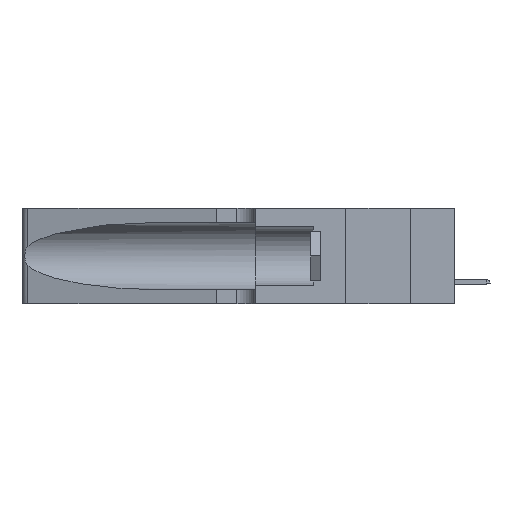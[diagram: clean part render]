
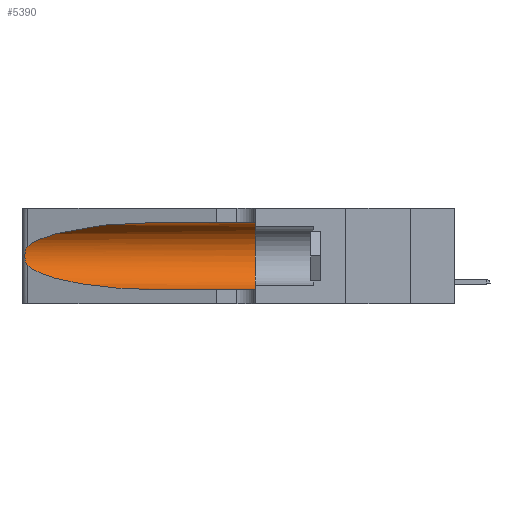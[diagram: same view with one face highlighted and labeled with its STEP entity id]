
A CAD part, left-side view. The second image highlights one B-rep face of the part: STEP entity #5390.
In plain terms, the highlighted cylindrical face has radius 3.308 mm (diameter 6.617 mm), a partial arc.
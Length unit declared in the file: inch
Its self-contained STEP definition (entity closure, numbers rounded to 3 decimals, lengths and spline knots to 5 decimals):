
#290 = CARTESIAN_POINT ( 'NONE',  ( 0.1305, 0.72297, 0.31525 ) ) ;
#758 = DIRECTION ( 'NONE',  ( 0., 0., 1. ) ) ;
#1511 = CARTESIAN_POINT ( 'NONE',  ( 0.25787, 1.23484, 0.2124 ) ) ;
#2479 = VERTEX_POINT ( 'NONE', #25399 ) ;
#2814 = DIRECTION ( 'NONE',  ( 0., -1., 0. ) ) ;
#3472 = DIRECTION ( 'NONE',  ( 0., 1., 0. ) ) ;
#3632 = ORIENTED_EDGE ( 'NONE', *, *, #14990, .T. ) ;
#4220 = CARTESIAN_POINT ( 'NONE',  ( 0.25856, 1.23593, 0.16098 ) ) ;
#5390 = ADVANCED_FACE ( 'NONE', ( #10882 ), #11783, .F. ) ;
#5573 = EDGE_LOOP ( 'NONE', ( #14647, #34118, #3632, #6699, #36847, #7488 ) ) ;
#5794 = LINE ( 'NONE', #29427, #13651 ) ;
#6699 = ORIENTED_EDGE ( 'NONE', *, *, #7355, .T. ) ;
#7143 = CARTESIAN_POINT ( 'NONE',  ( 0.26075, 1.23896, 0.19203 ) ) ;
#7355 = EDGE_CURVE ( 'NONE', #11016, #2479, #20298, .T. ) ;
#7488 = ORIENTED_EDGE ( 'NONE', *, *, #14777, .F. ) ;
#7536 = EDGE_CURVE ( 'NONE', #10165, #36781, #24513, .T. ) ;
#8660 = DIRECTION ( 'NONE',  ( 0., 0., -1. ) ) ;
#8939 = EDGE_CURVE ( 'NONE', #36781, #21660, #22074, .T. ) ;
#10009 = CARTESIAN_POINT ( 'NONE',  ( 0.25487, 1.22718, 0.22369 ) ) ;
#10065 = CARTESIAN_POINT ( 'NONE',  ( 0.26018, 1.23835, 0.19895 ) ) ;
#10165 = VERTEX_POINT ( 'NONE', #13570 ) ;
#10266 = CARTESIAN_POINT ( 'NONE',  ( 0.26017, 1.23833, 0.17102 ) ) ;
#10743 = CARTESIAN_POINT ( 'NONE',  ( 0.1305, 0.72297, 0.05475 ) ) ;
#10882 = FACE_OUTER_BOUND ( 'NONE', #5573, .T. ) ;
#11016 = VERTEX_POINT ( 'NONE', #10743 ) ;
#11783 = CYLINDRICAL_SURFACE ( 'NONE', #23109, 0.13025 ) ;
#12361 = CARTESIAN_POINT ( 'NONE',  ( 0.2373, 1.15595, 0.28018 ) ) ;
#13380 = CARTESIAN_POINT ( 'NONE',  ( 0.25555, 1.22993, 0.14849 ) ) ;
#13570 = CARTESIAN_POINT ( 'NONE',  ( 0.1305, 0.72297, 0.31525 ) ) ;
#13651 = VECTOR ( 'NONE', #14919, 39.37008 ) ;
#14504 = CARTESIAN_POINT ( 'NONE',  ( 0.1305, 1.61858, 0.05475 ) ) ;
#14647 = ORIENTED_EDGE ( 'NONE', *, *, #7536, .T. ) ;
#14688 = VERTEX_POINT ( 'NONE', #16323 ) ;
#14751 = CARTESIAN_POINT ( 'NONE',  ( 0.1305, 0.35, 0.185 ) ) ;
#14755 = AXIS2_PLACEMENT_3D ( 'NONE', #14751, #3472, #758 ) ;
#14777 = EDGE_CURVE ( 'NONE', #10165, #14688, #5794, .T. ) ;
#14919 = DIRECTION ( 'NONE',  ( 0., -1., 0. ) ) ;
#14990 = EDGE_CURVE ( 'NONE', #21660, #11016, #15143, .T. ) ;
#15109 = CARTESIAN_POINT ( 'NONE',  ( 0.25487, 1.22718, 0.22369 ) ) ;
#15143 =( BOUNDED_CURVE ( )  B_SPLINE_CURVE ( 3, ( #33874, #16657, #16080, #37141 ),
 .UNSPECIFIED., .F., .T. ) 
 B_SPLINE_CURVE_WITH_KNOTS ( ( 4, 4 ),
 ( 3.44316, 4.71239 ),
 .UNSPECIFIED. ) 
 CURVE ( )  GEOMETRIC_REPRESENTATION_ITEM ( )  RATIONAL_B_SPLINE_CURVE ( ( 1., 0.87, 0.87, 1. ) ) 
 REPRESENTATION_ITEM ( '' )  );
#16080 = CARTESIAN_POINT ( 'NONE',  ( 0.18966, 0.96281, 0.05475 ) ) ;
#16098 = CARTESIAN_POINT ( 'NONE',  ( 0.25487, 1.22718, 0.14631 ) ) ;
#16323 = CARTESIAN_POINT ( 'NONE',  ( 0.1305, 0.35, 0.31525 ) ) ;
#16657 = CARTESIAN_POINT ( 'NONE',  ( 0.2373, 1.15595, 0.08982 ) ) ;
#18933 = CARTESIAN_POINT ( 'NONE',  ( 0.18966, 0.96281, 0.31525 ) ) ;
#19383 = CARTESIAN_POINT ( 'NONE',  ( 0.25789, 1.23486, 0.15765 ) ) ;
#19882 = CARTESIAN_POINT ( 'NONE',  ( 0.25487, 1.22718, 0.14631 ) ) ;
#20254 = VECTOR ( 'NONE', #2814, 39.37008 ) ;
#20298 = LINE ( 'NONE', #14504, #20254 ) ;
#21132 = CARTESIAN_POINT ( 'NONE',  ( 0.25487, 1.22718, 0.22369 ) ) ;
#21660 = VERTEX_POINT ( 'NONE', #19882 ) ;
#22074 = B_SPLINE_CURVE_WITH_KNOTS ( 'NONE', 3,
 ( #21132, #29441, #30411, #1511, #36590, #10065, #7143, #33889, #10266, #4220, #19383, #30987, #13380, #16098 ),
 .UNSPECIFIED., .F., .F.,
 ( 4, 2, 2, 2, 2, 2, 4 ),
 ( 0., 0.00027, 0.00053, 0.00107, 0.0016, 0.00187, 0.00214 ),
 .UNSPECIFIED. ) ;
#23109 = AXIS2_PLACEMENT_3D ( 'NONE', #32901, #25603, #8660 ) ;
#24513 =( BOUNDED_CURVE ( )  B_SPLINE_CURVE ( 3, ( #290, #18933, #12361, #10009 ),
 .UNSPECIFIED., .F., .T. ) 
 B_SPLINE_CURVE_WITH_KNOTS ( ( 4, 4 ),
 ( 1.5708, 2.84003 ),
 .UNSPECIFIED. ) 
 CURVE ( )  GEOMETRIC_REPRESENTATION_ITEM ( )  RATIONAL_B_SPLINE_CURVE ( ( 1., 0.87, 0.87, 1. ) ) 
 REPRESENTATION_ITEM ( '' )  );
#24647 = EDGE_CURVE ( 'NONE', #14688, #2479, #36991, .T. ) ;
#25399 = CARTESIAN_POINT ( 'NONE',  ( 0.1305, 0.35, 0.05475 ) ) ;
#25603 = DIRECTION ( 'NONE',  ( 0., -1., 0. ) ) ;
#29427 = CARTESIAN_POINT ( 'NONE',  ( 0.1305, 1.61858, 0.31525 ) ) ;
#29441 = CARTESIAN_POINT ( 'NONE',  ( 0.25555, 1.22994, 0.2215 ) ) ;
#30411 = CARTESIAN_POINT ( 'NONE',  ( 0.25639, 1.23184, 0.21858 ) ) ;
#30987 = CARTESIAN_POINT ( 'NONE',  ( 0.25639, 1.23186, 0.15144 ) ) ;
#32901 = CARTESIAN_POINT ( 'NONE',  ( 0.1305, 1.61858, 0.185 ) ) ;
#33874 = CARTESIAN_POINT ( 'NONE',  ( 0.25487, 1.22718, 0.14631 ) ) ;
#33889 = CARTESIAN_POINT ( 'NONE',  ( 0.26075, 1.23896, 0.178 ) ) ;
#34118 = ORIENTED_EDGE ( 'NONE', *, *, #8939, .T. ) ;
#36590 = CARTESIAN_POINT ( 'NONE',  ( 0.25854, 1.2359, 0.20912 ) ) ;
#36781 = VERTEX_POINT ( 'NONE', #15109 ) ;
#36847 = ORIENTED_EDGE ( 'NONE', *, *, #24647, .F. ) ;
#36991 = CIRCLE ( 'NONE', #14755, 0.13025 ) ;
#37141 = CARTESIAN_POINT ( 'NONE',  ( 0.1305, 0.72297, 0.05475 ) ) ;
